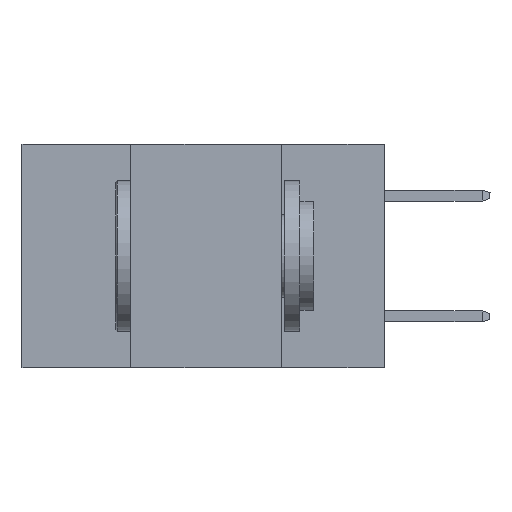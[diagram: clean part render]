
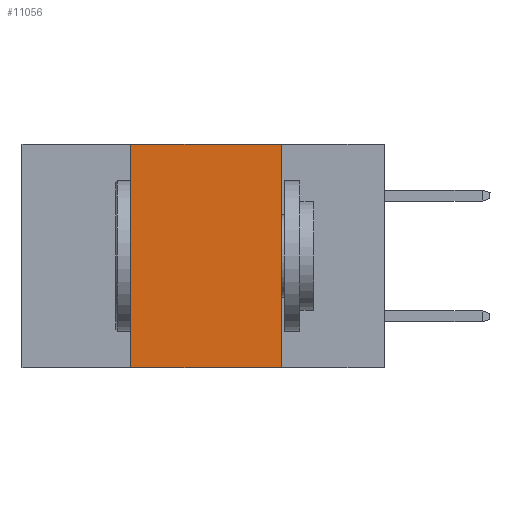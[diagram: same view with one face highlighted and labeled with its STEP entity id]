
A CAD part, left-side view. The second image highlights one B-rep face of the part: STEP entity #11056.
In plain terms, the highlighted planar face has unit normal (-1, 0, 0).
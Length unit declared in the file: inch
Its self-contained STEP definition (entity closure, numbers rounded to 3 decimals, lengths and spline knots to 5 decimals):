
#16 = VERTEX_POINT ( 'NONE', #4373 ) ;
#37 = DIRECTION ( 'NONE',  ( 0., -1., 0. ) ) ;
#47 = VERTEX_POINT ( 'NONE', #2898 ) ;
#122 = CARTESIAN_POINT ( 'NONE',  ( 0., 0.6, -0.37 ) ) ;
#588 = CARTESIAN_POINT ( 'NONE',  ( 0., 0.42, 0. ) ) ;
#1838 = VECTOR ( 'NONE', #8554, 39.37008 ) ;
#2808 = CARTESIAN_POINT ( 'NONE',  ( 0., 0.6, 0. ) ) ;
#2898 = CARTESIAN_POINT ( 'NONE',  ( 0., 0.17, -0.37 ) ) ;
#2947 = DIRECTION ( 'NONE',  ( 0., 0., -1. ) ) ;
#3098 = ORIENTED_EDGE ( 'NONE', *, *, #12095, .F. ) ;
#3127 = LINE ( 'NONE', #122, #3839 ) ;
#3377 = VERTEX_POINT ( 'NONE', #4168 ) ;
#3839 = VECTOR ( 'NONE', #37, 39.37008 ) ;
#4168 = CARTESIAN_POINT ( 'NONE',  ( 0., 0.17, 0. ) ) ;
#4275 = CARTESIAN_POINT ( 'NONE',  ( 0., 0.6, 0. ) ) ;
#4307 = LINE ( 'NONE', #2808, #1838 ) ;
#4373 = CARTESIAN_POINT ( 'NONE',  ( 0., 0.42, 0. ) ) ;
#4522 = AXIS2_PLACEMENT_3D ( 'NONE', #4275, #7064, #6032 ) ;
#4679 = EDGE_LOOP ( 'NONE', ( #7447, #7545, #3098, #8743 ) ) ;
#4708 = VECTOR ( 'NONE', #6881, 39.37008 ) ;
#6032 = DIRECTION ( 'NONE',  ( 0., 0., -1. ) ) ;
#6137 = CARTESIAN_POINT ( 'NONE',  ( 0., 0.42, -0.37 ) ) ;
#6385 = LINE ( 'NONE', #7486, #12110 ) ;
#6881 = DIRECTION ( 'NONE',  ( 0., 0., 1. ) ) ;
#7008 = EDGE_CURVE ( 'NONE', #3377, #47, #6385, .T. ) ;
#7064 = DIRECTION ( 'NONE',  ( 1., 0., 0. ) ) ;
#7447 = ORIENTED_EDGE ( 'NONE', *, *, #7008, .F. ) ;
#7486 = CARTESIAN_POINT ( 'NONE',  ( 0., 0.17, 0. ) ) ;
#7545 = ORIENTED_EDGE ( 'NONE', *, *, #7986, .F. ) ;
#7986 = EDGE_CURVE ( 'NONE', #16, #3377, #4307, .T. ) ;
#8554 = DIRECTION ( 'NONE',  ( 0., -1., 0. ) ) ;
#8629 = VERTEX_POINT ( 'NONE', #6137 ) ;
#8743 = ORIENTED_EDGE ( 'NONE', *, *, #11329, .T. ) ;
#8855 = PLANE ( 'NONE',  #4522 ) ;
#9575 = LINE ( 'NONE', #588, #4708 ) ;
#10457 = FACE_OUTER_BOUND ( 'NONE', #4679, .T. ) ;
#11056 = ADVANCED_FACE ( 'NONE', ( #10457 ), #8855, .F. ) ;
#11329 = EDGE_CURVE ( 'NONE', #8629, #47, #3127, .T. ) ;
#12095 = EDGE_CURVE ( 'NONE', #8629, #16, #9575, .T. ) ;
#12110 = VECTOR ( 'NONE', #2947, 39.37008 ) ;
